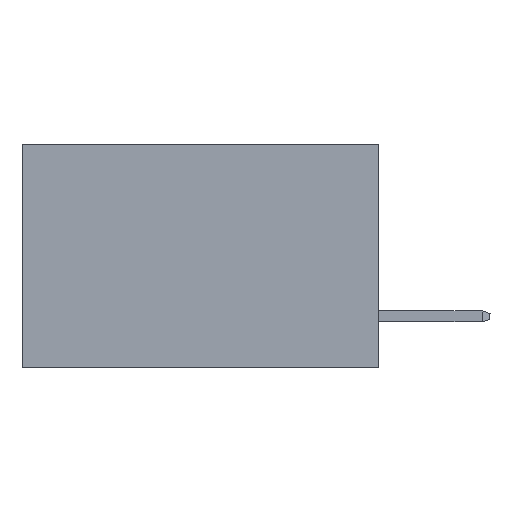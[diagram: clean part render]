
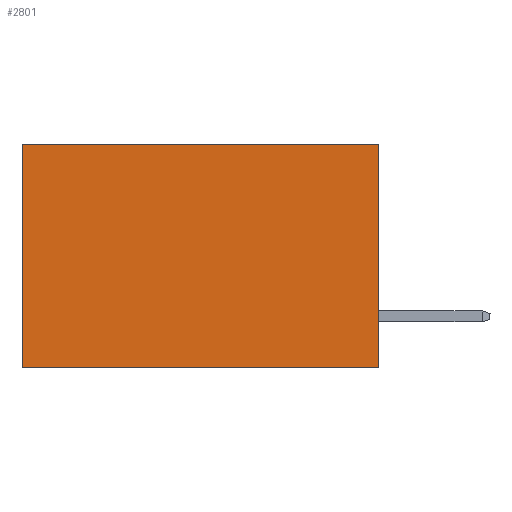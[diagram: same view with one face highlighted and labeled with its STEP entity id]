
A CAD part, left-side view. The second image highlights one B-rep face of the part: STEP entity #2801.
In plain terms, the highlighted planar face has unit normal (-1, 0, 0).
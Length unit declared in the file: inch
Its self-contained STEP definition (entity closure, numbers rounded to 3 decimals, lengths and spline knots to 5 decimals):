
#117 = VECTOR ( 'NONE', #14797, 39.37008 ) ;
#260 = VERTEX_POINT ( 'NONE', #10995 ) ;
#329 = CARTESIAN_POINT ( 'NONE',  ( 0.277, 0., 0. ) ) ;
#585 = LINE ( 'NONE', #2833, #117 ) ;
#899 = VERTEX_POINT ( 'NONE', #10445 ) ;
#1019 = DIRECTION ( 'NONE',  ( 0., 0., -1. ) ) ;
#1113 = EDGE_CURVE ( 'NONE', #899, #260, #12396, .T. ) ;
#1923 = DIRECTION ( 'NONE',  ( 0., 0., -1. ) ) ;
#2337 = ORIENTED_EDGE ( 'NONE', *, *, #1113, .T. ) ;
#2508 = FACE_OUTER_BOUND ( 'NONE', #9889, .T. ) ;
#2801 = ADVANCED_FACE ( 'NONE', ( #2508 ), #8001, .F. ) ;
#2833 = CARTESIAN_POINT ( 'NONE',  ( 0.277, 0., -0.37 ) ) ;
#3393 = CARTESIAN_POINT ( 'NONE',  ( 0.277, 0., -0.37 ) ) ;
#3804 = DIRECTION ( 'NONE',  ( 1., 0., 0. ) ) ;
#4724 = DIRECTION ( 'NONE',  ( 0., 1., 0. ) ) ;
#5305 = VECTOR ( 'NONE', #4724, 39.37008 ) ;
#6257 = DIRECTION ( 'NONE',  ( 0., 1., 0. ) ) ;
#6665 = LINE ( 'NONE', #16813, #13355 ) ;
#6772 = EDGE_CURVE ( 'NONE', #899, #17154, #585, .T. ) ;
#7085 = EDGE_CURVE ( 'NONE', #17154, #11510, #9377, .T. ) ;
#8001 = PLANE ( 'NONE',  #14755 ) ;
#9270 = VECTOR ( 'NONE', #6257, 39.37008 ) ;
#9377 = LINE ( 'NONE', #11461, #5305 ) ;
#9399 = ORIENTED_EDGE ( 'NONE', *, *, #6772, .F. ) ;
#9889 = EDGE_LOOP ( 'NONE', ( #14861, #12745, #9399, #2337 ) ) ;
#10445 = CARTESIAN_POINT ( 'NONE',  ( 0.277, 0., 0. ) ) ;
#10995 = CARTESIAN_POINT ( 'NONE',  ( 0.277, 0.59, 0. ) ) ;
#11461 = CARTESIAN_POINT ( 'NONE',  ( 0.277, 0., -0.37 ) ) ;
#11510 = VERTEX_POINT ( 'NONE', #12464 ) ;
#11951 = EDGE_CURVE ( 'NONE', #260, #11510, #6665, .T. ) ;
#12396 = LINE ( 'NONE', #329, #9270 ) ;
#12464 = CARTESIAN_POINT ( 'NONE',  ( 0.277, 0.59, -0.37 ) ) ;
#12745 = ORIENTED_EDGE ( 'NONE', *, *, #7085, .F. ) ;
#12885 = CARTESIAN_POINT ( 'NONE',  ( 0.277, 0., -0.37 ) ) ;
#13355 = VECTOR ( 'NONE', #1019, 39.37008 ) ;
#14755 = AXIS2_PLACEMENT_3D ( 'NONE', #3393, #3804, #1923 ) ;
#14797 = DIRECTION ( 'NONE',  ( 0., 0., -1. ) ) ;
#14861 = ORIENTED_EDGE ( 'NONE', *, *, #11951, .T. ) ;
#16813 = CARTESIAN_POINT ( 'NONE',  ( 0.277, 0.59, -0.37 ) ) ;
#17154 = VERTEX_POINT ( 'NONE', #12885 ) ;
